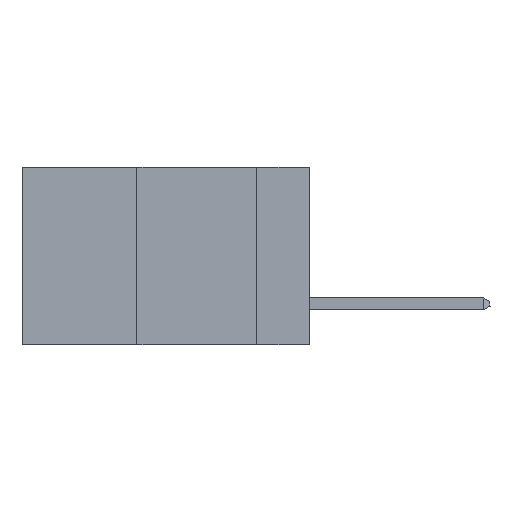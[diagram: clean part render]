
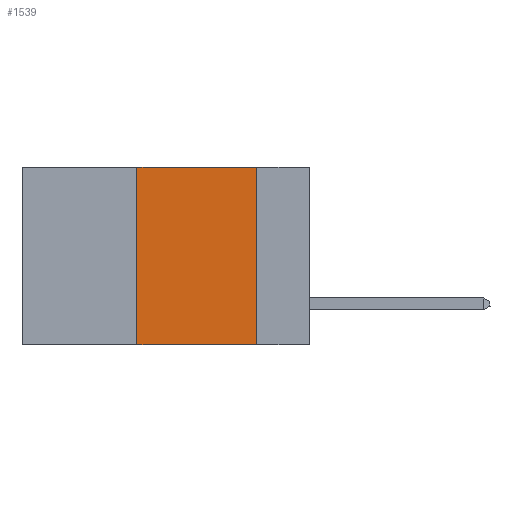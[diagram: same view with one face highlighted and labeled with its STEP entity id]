
A CAD part, left-side view. The second image highlights one B-rep face of the part: STEP entity #1539.
In plain terms, the highlighted planar face has unit normal (-1, 0, 0).
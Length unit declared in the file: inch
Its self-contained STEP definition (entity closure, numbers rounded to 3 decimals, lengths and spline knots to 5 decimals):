
#384 = EDGE_CURVE ( 'NONE', #10970, #9378, #3872, .T. ) ;
#535 = CARTESIAN_POINT ( 'NONE',  ( 0., 0.6, 0. ) ) ;
#998 = VECTOR ( 'NONE', #14628, 39.37008 ) ;
#1321 = EDGE_LOOP ( 'NONE', ( #11404, #7995, #9403, #13645 ) ) ;
#1539 = ADVANCED_FACE ( 'NONE', ( #4681 ), #7188, .F. ) ;
#2297 = EDGE_CURVE ( 'NONE', #10970, #3791, #12180, .T. ) ;
#3791 = VERTEX_POINT ( 'NONE', #9471 ) ;
#3872 = LINE ( 'NONE', #7922, #998 ) ;
#4681 = FACE_OUTER_BOUND ( 'NONE', #1321, .T. ) ;
#6015 = EDGE_CURVE ( 'NONE', #9384, #9378, #7319, .T. ) ;
#6023 = DIRECTION ( 'NONE',  ( 0., 0., 1. ) ) ;
#6626 = CARTESIAN_POINT ( 'NONE',  ( 0., 0.6, 0. ) ) ;
#6791 = DIRECTION ( 'NONE',  ( 0., -1., 0. ) ) ;
#7188 = PLANE ( 'NONE',  #15638 ) ;
#7298 = CARTESIAN_POINT ( 'NONE',  ( 0., 0.36, 0. ) ) ;
#7319 = LINE ( 'NONE', #10349, #9166 ) ;
#7473 = EDGE_CURVE ( 'NONE', #3791, #9384, #13083, .T. ) ;
#7922 = CARTESIAN_POINT ( 'NONE',  ( 0., 0.6, -0.37 ) ) ;
#7995 = ORIENTED_EDGE ( 'NONE', *, *, #7473, .F. ) ;
#8110 = CARTESIAN_POINT ( 'NONE',  ( 0., 0.11, -0.37 ) ) ;
#8682 = VECTOR ( 'NONE', #6023, 39.37008 ) ;
#9166 = VECTOR ( 'NONE', #11665, 39.37008 ) ;
#9378 = VERTEX_POINT ( 'NONE', #8110 ) ;
#9384 = VERTEX_POINT ( 'NONE', #12058 ) ;
#9403 = ORIENTED_EDGE ( 'NONE', *, *, #2297, .F. ) ;
#9471 = CARTESIAN_POINT ( 'NONE',  ( 0., 0.36, 0. ) ) ;
#9610 = VECTOR ( 'NONE', #6791, 39.37008 ) ;
#9711 = CARTESIAN_POINT ( 'NONE',  ( 0., 0.36, -0.37 ) ) ;
#10349 = CARTESIAN_POINT ( 'NONE',  ( 0., 0.11, 0. ) ) ;
#10970 = VERTEX_POINT ( 'NONE', #9711 ) ;
#11404 = ORIENTED_EDGE ( 'NONE', *, *, #6015, .F. ) ;
#11665 = DIRECTION ( 'NONE',  ( 0., 0., -1. ) ) ;
#12058 = CARTESIAN_POINT ( 'NONE',  ( 0., 0.11, 0. ) ) ;
#12180 = LINE ( 'NONE', #7298, #8682 ) ;
#13083 = LINE ( 'NONE', #6626, #9610 ) ;
#13541 = DIRECTION ( 'NONE',  ( 0., 0., -1. ) ) ;
#13645 = ORIENTED_EDGE ( 'NONE', *, *, #384, .T. ) ;
#14628 = DIRECTION ( 'NONE',  ( 0., -1., 0. ) ) ;
#14794 = DIRECTION ( 'NONE',  ( 1., 0., 0. ) ) ;
#15638 = AXIS2_PLACEMENT_3D ( 'NONE', #535, #14794, #13541 ) ;
